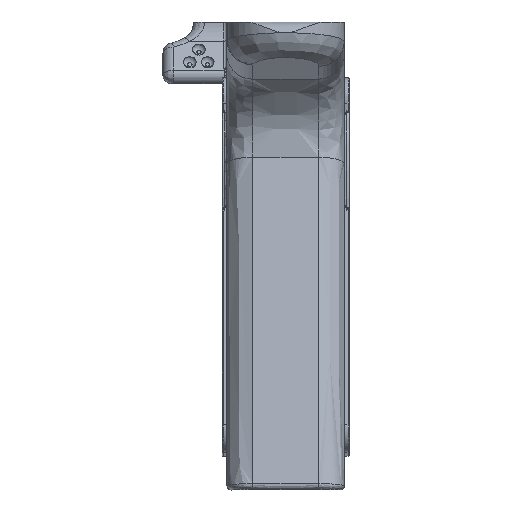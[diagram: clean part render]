
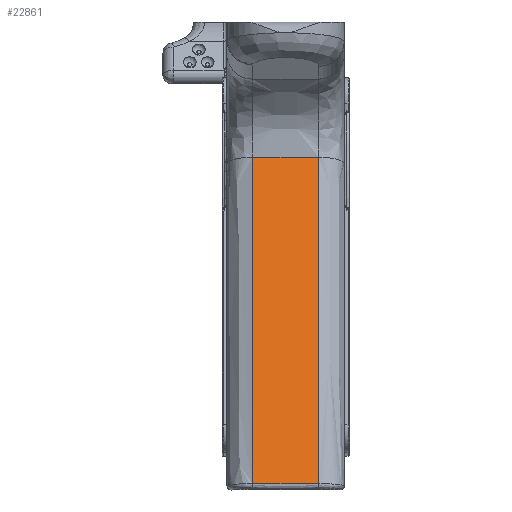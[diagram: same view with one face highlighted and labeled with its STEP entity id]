
A CAD part, front view. The second image highlights one B-rep face of the part: STEP entity #22861.
In plain terms, the highlighted free-form (B-spline) face has degree [5, 1] with [25, 2] control points.
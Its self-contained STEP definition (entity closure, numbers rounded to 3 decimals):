
#750=(
BOUNDED_SURFACE()
B_SPLINE_SURFACE(5,1,((#31950,#31951),(#31952,#31953),(#31954,#31955),(#31956,
#31957),(#31958,#31959),(#31960,#31961),(#31962,#31963),(#31964,#31965),
(#31966,#31967),(#31968,#31969),(#31970,#31971),(#31972,#31973),(#31974,
#31975),(#31976,#31977),(#31978,#31979),(#31980,#31981),(#31982,#31983),
(#31984,#31985),(#31986,#31987),(#31988,#31989),(#31990,#31991),(#31992,
#31993),(#31994,#31995),(#31996,#31997),(#31998,#31999)),.UNSPECIFIED.,
 .F.,.F.,.F.)
B_SPLINE_SURFACE_WITH_KNOTS((6,5,1,1,1,1,1,1,1,1,1,5,6),(2,2),(-1.178,
-1.,-0.9,-0.8,-0.7,-0.6,-0.5,-0.4,-0.3,-0.2,-0.1,0.,2.179),(-2.379,
5.132),.UNSPECIFIED.)
GEOMETRIC_REPRESENTATION_ITEM()
RATIONAL_B_SPLINE_SURFACE(((1.,1.),(1.,1.),(1.,1.),(1.,1.),(1.,1.),(1.,
1.),(1.,1.),(1.,1.),(1.,1.),(1.,1.),(1.,1.),(1.,1.),(1.,1.),(1.,1.),(1.,
1.),(1.,1.),(1.,1.),(1.,1.),(1.,1.),(1.,1.),(1.,1.),(1.,1.),(1.,1.),(1.,
1.),(1.,1.)))
REPRESENTATION_ITEM('')
SURFACE()
);
#1720=B_SPLINE_CURVE_WITH_KNOTS('',3,(#30573,#30574,#30575,#30576,#30577,
#30578),.UNSPECIFIED.,.F.,.F.,(4,2,4),(-7.954,-0.629,
0.),.UNSPECIFIED.);
#1731=B_SPLINE_CURVE_WITH_KNOTS('',3,(#30865,#30866,#30867,#30868,#30869,
#30870,#30871),.UNSPECIFIED.,.F.,.F.,(4,2,1,4),(-7.954,-7.325,
-3.139,0.),.UNSPECIFIED.);
#1809=B_SPLINE_CURVE_WITH_KNOTS('',3,(#31942,#31943,#31944,#31945),
 .UNSPECIFIED.,.F.,.F.,(4,4),(0.6,2.145),.UNSPECIFIED.);
#2735=FACE_OUTER_BOUND('',#4132,.T.);
#4132=EDGE_LOOP('',(#15635,#15636,#15637,#15638));
#5532=LINE('',#30471,#7133);
#7133=VECTOR('',#25723,10.);
#9338=VERTEX_POINT('',#30343);
#9346=VERTEX_POINT('',#30470);
#9348=VERTEX_POINT('',#30572);
#9387=VERTEX_POINT('',#30863);
#11656=EDGE_CURVE('',#9338,#9346,#5532,.T.);
#11660=EDGE_CURVE('',#9346,#9348,#1720,.T.);
#11713=EDGE_CURVE('',#9387,#9338,#1731,.T.);
#11924=EDGE_CURVE('',#9348,#9387,#1809,.T.);
#15635=ORIENTED_EDGE('',*,*,#11660,.F.);
#15636=ORIENTED_EDGE('',*,*,#11656,.F.);
#15637=ORIENTED_EDGE('',*,*,#11713,.F.);
#15638=ORIENTED_EDGE('',*,*,#11924,.F.);
#22861=ADVANCED_FACE('',(#2735),#750,.F.);
#25723=DIRECTION('',(1.,0.,0.));
#30343=CARTESIAN_POINT('',(0.725,-90.162,100.53));
#30470=CARTESIAN_POINT('',(16.175,-90.162,100.53));
#30471=CARTESIAN_POINT('',(22.175,-90.162,100.53));
#30572=CARTESIAN_POINT('',(16.175,-68.765,24.118));
#30573=CARTESIAN_POINT('Ctrl Pts',(16.175,-90.162,100.53));
#30574=CARTESIAN_POINT('Ctrl Pts',(16.175,-83.279,77.132));
#30575=CARTESIAN_POINT('Ctrl Pts',(16.175,-76.502,53.727));
#30576=CARTESIAN_POINT('Ctrl Pts',(16.175,-69.825,28.185));
#30577=CARTESIAN_POINT('Ctrl Pts',(16.175,-69.294,26.148));
#30578=CARTESIAN_POINT('Ctrl Pts',(16.175,-68.765,24.118));
#30863=CARTESIAN_POINT('',(0.725,-68.765,24.118));
#30865=CARTESIAN_POINT('Ctrl Pts',(0.725,-68.765,24.118));
#30866=CARTESIAN_POINT('Ctrl Pts',(0.725,-69.294,
26.148));
#30867=CARTESIAN_POINT('Ctrl Pts',(0.725,-69.824,
28.178));
#30868=CARTESIAN_POINT('Ctrl Pts',(0.725,-73.858,
43.642));
#30869=CARTESIAN_POINT('Ctrl Pts',(0.725,-80.386,
67.092));
#30870=CARTESIAN_POINT('Ctrl Pts',(0.725,-87.212,
90.502));
#30871=CARTESIAN_POINT('Ctrl Pts',(0.725,-90.162,
100.53));
#31942=CARTESIAN_POINT('Ctrl Pts',(16.175,-68.765,24.118));
#31943=CARTESIAN_POINT('Ctrl Pts',(11.025,-68.765,24.118));
#31944=CARTESIAN_POINT('Ctrl Pts',(5.875,-68.765,24.118));
#31945=CARTESIAN_POINT('Ctrl Pts',(0.725,-68.765,24.118));
#31950=CARTESIAN_POINT('Ctrl Pts',(45.968,-95.649,119.15));
#31951=CARTESIAN_POINT('Ctrl Pts',(-29.15,-95.649,
119.15));
#31952=CARTESIAN_POINT('Ctrl Pts',(45.968,-94.719,115.995));
#31953=CARTESIAN_POINT('Ctrl Pts',(-29.15,-94.719,
115.995));
#31954=CARTESIAN_POINT('Ctrl Pts',(45.968,-93.789,112.841));
#31955=CARTESIAN_POINT('Ctrl Pts',(-29.15,-93.789,112.841));
#31956=CARTESIAN_POINT('Ctrl Pts',(45.968,-92.86,109.686));
#31957=CARTESIAN_POINT('Ctrl Pts',(-29.15,-92.86,
109.686));
#31958=CARTESIAN_POINT('Ctrl Pts',(45.968,-91.93,106.531));
#31959=CARTESIAN_POINT('Ctrl Pts',(-29.15,-91.93,
106.531));
#31960=CARTESIAN_POINT('Ctrl Pts',(45.968,-91.,103.376));
#31961=CARTESIAN_POINT('Ctrl Pts',(-29.15,-91.,
103.376));
#31962=CARTESIAN_POINT('Ctrl Pts',(45.968,-90.477,101.6));
#31963=CARTESIAN_POINT('Ctrl Pts',(-29.15,-90.477,
101.6));
#31964=CARTESIAN_POINT('Ctrl Pts',(45.968,-89.439,98.075));
#31965=CARTESIAN_POINT('Ctrl Pts',(-29.15,-89.439,
98.075));
#31966=CARTESIAN_POINT('Ctrl Pts',(45.968,-87.911,92.865));
#31967=CARTESIAN_POINT('Ctrl Pts',(-29.15,-87.911,
92.865));
#31968=CARTESIAN_POINT('Ctrl Pts',(45.968,-85.928,86.075));
#31969=CARTESIAN_POINT('Ctrl Pts',(-29.15,-85.928,
86.075));
#31970=CARTESIAN_POINT('Ctrl Pts',(45.968,-83.55,77.871));
#31971=CARTESIAN_POINT('Ctrl Pts',(-29.15,-83.55,
77.871));
#31972=CARTESIAN_POINT('Ctrl Pts',(45.968,-81.281,69.978));
#31973=CARTESIAN_POINT('Ctrl Pts',(-29.15,-81.281,
69.978));
#31974=CARTESIAN_POINT('Ctrl Pts',(45.968,-79.134,62.429));
#31975=CARTESIAN_POINT('Ctrl Pts',(-29.15,-79.134,
62.429));
#31976=CARTESIAN_POINT('Ctrl Pts',(45.968,-77.12,55.253));
#31977=CARTESIAN_POINT('Ctrl Pts',(-29.15,-77.12,
55.253));
#31978=CARTESIAN_POINT('Ctrl Pts',(45.968,-75.239,48.457));
#31979=CARTESIAN_POINT('Ctrl Pts',(-29.15,-75.239,
48.457));
#31980=CARTESIAN_POINT('Ctrl Pts',(45.968,-73.485,42.019));
#31981=CARTESIAN_POINT('Ctrl Pts',(-29.15,-73.485,
42.019));
#31982=CARTESIAN_POINT('Ctrl Pts',(45.968,-72.177,37.138));
#31983=CARTESIAN_POINT('Ctrl Pts',(-29.15,-72.177,
37.138));
#31984=CARTESIAN_POINT('Ctrl Pts',(45.968,-71.246,33.618));
#31985=CARTESIAN_POINT('Ctrl Pts',(-29.15,-71.246,33.618));
#31986=CARTESIAN_POINT('Ctrl Pts',(45.968,-70.647,31.334));
#31987=CARTESIAN_POINT('Ctrl Pts',(-29.15,-70.647,
31.334));
#31988=CARTESIAN_POINT('Ctrl Pts',(45.968,-70.353,30.208));
#31989=CARTESIAN_POINT('Ctrl Pts',(-29.15,-70.353,
30.208));
#31990=CARTESIAN_POINT('Ctrl Pts',(45.968,-63.949,5.658));
#31991=CARTESIAN_POINT('Ctrl Pts',(-29.15,-63.949,
5.658));
#31992=CARTESIAN_POINT('Ctrl Pts',(45.968,-57.545,-18.892));
#31993=CARTESIAN_POINT('Ctrl Pts',(-29.15,-57.545,
-18.892));
#31994=CARTESIAN_POINT('Ctrl Pts',(45.968,-51.14,-43.442));
#31995=CARTESIAN_POINT('Ctrl Pts',(-29.15,-51.14,
-43.442));
#31996=CARTESIAN_POINT('Ctrl Pts',(45.968,-44.736,-67.992));
#31997=CARTESIAN_POINT('Ctrl Pts',(-29.15,-44.736,
-67.992));
#31998=CARTESIAN_POINT('Ctrl Pts',(45.968,-38.332,-92.542));
#31999=CARTESIAN_POINT('Ctrl Pts',(-29.15,-38.332,-92.542));
